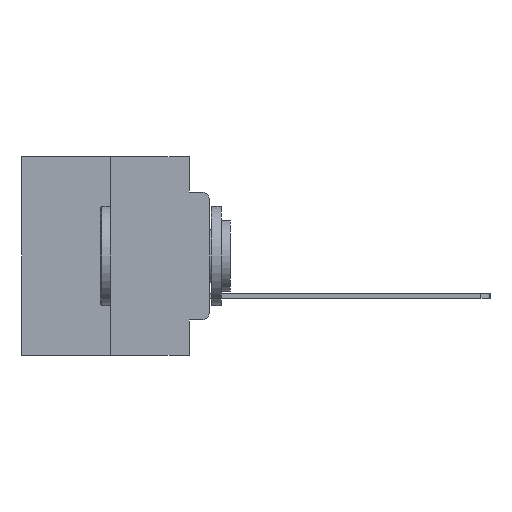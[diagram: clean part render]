
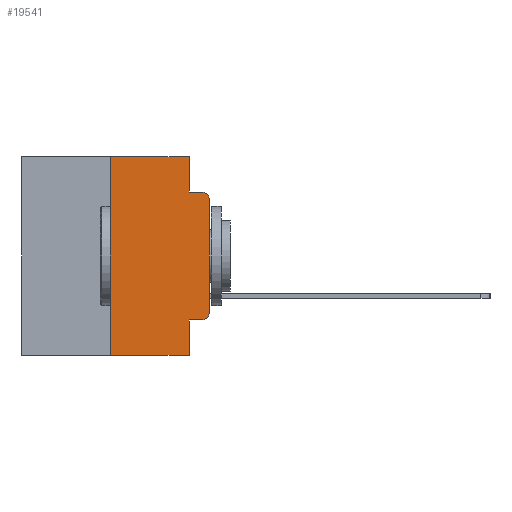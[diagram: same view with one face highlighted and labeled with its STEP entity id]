
A CAD part, left-side view. The second image highlights one B-rep face of the part: STEP entity #19541.
In plain terms, the highlighted planar face has unit normal (-1, 0, 0).
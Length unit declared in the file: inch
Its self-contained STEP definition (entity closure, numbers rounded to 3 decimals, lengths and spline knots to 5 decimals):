
#303 = VECTOR ( 'NONE', #25448, 39.37008 ) ;
#436 = CARTESIAN_POINT ( 'NONE',  ( 0., 0.473, 0. ) ) ;
#485 = ORIENTED_EDGE ( 'NONE', *, *, #19054, .T. ) ;
#502 = CARTESIAN_POINT ( 'NONE',  ( 0., 0.051, 0. ) ) ;
#745 = CARTESIAN_POINT ( 'NONE',  ( 0., 0.473, -0.5 ) ) ;
#862 = AXIS2_PLACEMENT_3D ( 'NONE', #10973, #25536, #13118 ) ;
#1314 = EDGE_CURVE ( 'NONE', #26206, #25900, #19107, .T. ) ;
#1725 = ORIENTED_EDGE ( 'NONE', *, *, #19400, .F. ) ;
#2042 = AXIS2_PLACEMENT_3D ( 'NONE', #21464, #8887, #23537 ) ;
#2920 = DIRECTION ( 'NONE',  ( 0., -1., 0. ) ) ;
#3387 = VECTOR ( 'NONE', #6915, 39.37008 ) ;
#3473 = CARTESIAN_POINT ( 'NONE',  ( 0., 0.051, -0.0885 ) ) ;
#3504 = VECTOR ( 'NONE', #16358, 39.37008 ) ;
#3799 = EDGE_CURVE ( 'NONE', #7085, #5451, #5358, .T. ) ;
#4054 = ORIENTED_EDGE ( 'NONE', *, *, #3799, .T. ) ;
#4371 = CARTESIAN_POINT ( 'NONE',  ( 0., 0.051, -0.4115 ) ) ;
#4598 = VERTEX_POINT ( 'NONE', #15596 ) ;
#5358 = LINE ( 'NONE', #16427, #16022 ) ;
#5361 = CIRCLE ( 'NONE', #862, 0.02 ) ;
#5451 = VERTEX_POINT ( 'NONE', #12956 ) ;
#6039 = VERTEX_POINT ( 'NONE', #6753 ) ;
#6254 = ORIENTED_EDGE ( 'NONE', *, *, #1314, .F. ) ;
#6753 = CARTESIAN_POINT ( 'NONE',  ( 0., 0.051, -0.0885 ) ) ;
#6915 = DIRECTION ( 'NONE',  ( 0., -1., 0. ) ) ;
#7085 = VERTEX_POINT ( 'NONE', #4371 ) ;
#8029 = VECTOR ( 'NONE', #9062, 39.37008 ) ;
#8144 = CARTESIAN_POINT ( 'NONE',  ( 0., 0.25, 0. ) ) ;
#8887 = DIRECTION ( 'NONE',  ( -1., 0., 0. ) ) ;
#9062 = DIRECTION ( 'NONE',  ( 0., 0., -1. ) ) ;
#9314 = LINE ( 'NONE', #745, #19206 ) ;
#9753 = LINE ( 'NONE', #436, #3387 ) ;
#9881 = EDGE_CURVE ( 'NONE', #4598, #6039, #19247, .T. ) ;
#9950 = CARTESIAN_POINT ( 'NONE',  ( 0., 0.02, -0.0885 ) ) ;
#10298 = VERTEX_POINT ( 'NONE', #17089 ) ;
#10390 = DIRECTION ( 'NONE',  ( 0., 0., -1. ) ) ;
#10875 = CARTESIAN_POINT ( 'NONE',  ( 0., 0., 0. ) ) ;
#10952 = ORIENTED_EDGE ( 'NONE', *, *, #19436, .F. ) ;
#10973 = CARTESIAN_POINT ( 'NONE',  ( 0., 0.02, -0.3915 ) ) ;
#11281 = CARTESIAN_POINT ( 'NONE',  ( 0., 0.25, -0.5 ) ) ;
#12907 = EDGE_CURVE ( 'NONE', #27122, #15659, #14839, .T. ) ;
#12956 = CARTESIAN_POINT ( 'NONE',  ( 0., 0.02, -0.4115 ) ) ;
#13118 = DIRECTION ( 'NONE',  ( 0., 0., -1. ) ) ;
#13703 = VECTOR ( 'NONE', #26496, 39.37008 ) ;
#14209 = EDGE_CURVE ( 'NONE', #26206, #10298, #9314, .T. ) ;
#14231 = CARTESIAN_POINT ( 'NONE',  ( 0., 0.051, 0. ) ) ;
#14839 = CIRCLE ( 'NONE', #2042, 0.02 ) ;
#15596 = CARTESIAN_POINT ( 'NONE',  ( 0., 0.051, 0. ) ) ;
#15659 = VERTEX_POINT ( 'NONE', #9950 ) ;
#16022 = VECTOR ( 'NONE', #24745, 39.37008 ) ;
#16358 = DIRECTION ( 'NONE',  ( 0., 0., 1. ) ) ;
#16427 = CARTESIAN_POINT ( 'NONE',  ( 0., 0.051, -0.4115 ) ) ;
#16537 = VERTEX_POINT ( 'NONE', #17227 ) ;
#16683 = CARTESIAN_POINT ( 'NONE',  ( 0., 0.473, 0. ) ) ;
#17089 = CARTESIAN_POINT ( 'NONE',  ( 0., 0.051, -0.5 ) ) ;
#17227 = CARTESIAN_POINT ( 'NONE',  ( 0., 0., -0.3915 ) ) ;
#17430 = CARTESIAN_POINT ( 'NONE',  ( 0., 0.25, 0. ) ) ;
#18614 = VECTOR ( 'NONE', #26595, 39.37008 ) ;
#18928 = ORIENTED_EDGE ( 'NONE', *, *, #12907, .T. ) ;
#19054 = EDGE_CURVE ( 'NONE', #16537, #27122, #22207, .T. ) ;
#19086 = EDGE_CURVE ( 'NONE', #5451, #16537, #5361, .T. ) ;
#19107 = LINE ( 'NONE', #17430, #3504 ) ;
#19206 = VECTOR ( 'NONE', #2920, 39.37008 ) ;
#19247 = LINE ( 'NONE', #502, #8029 ) ;
#19268 = LINE ( 'NONE', #3473, #13703 ) ;
#19400 = EDGE_CURVE ( 'NONE', #6039, #15659, #19268, .T. ) ;
#19436 = EDGE_CURVE ( 'NONE', #7085, #10298, #24106, .T. ) ;
#19541 = ADVANCED_FACE ( 'NONE', ( #26308 ), #20892, .F. ) ;
#19806 = EDGE_CURVE ( 'NONE', #25900, #4598, #9753, .T. ) ;
#20823 = ORIENTED_EDGE ( 'NONE', *, *, #14209, .T. ) ;
#20892 = PLANE ( 'NONE',  #23026 ) ;
#21240 = EDGE_LOOP ( 'NONE', ( #485, #18928, #1725, #22002, #23304, #6254, #20823, #10952, #4054, #23651 ) ) ;
#21464 = CARTESIAN_POINT ( 'NONE',  ( 0., 0.02, -0.1085 ) ) ;
#22002 = ORIENTED_EDGE ( 'NONE', *, *, #9881, .F. ) ;
#22207 = LINE ( 'NONE', #10875, #303 ) ;
#22953 = DIRECTION ( 'NONE',  ( 1., 0., 0. ) ) ;
#23026 = AXIS2_PLACEMENT_3D ( 'NONE', #16683, #22953, #10390 ) ;
#23304 = ORIENTED_EDGE ( 'NONE', *, *, #19806, .F. ) ;
#23537 = DIRECTION ( 'NONE',  ( 0., 0., -1. ) ) ;
#23651 = ORIENTED_EDGE ( 'NONE', *, *, #19086, .T. ) ;
#24106 = LINE ( 'NONE', #14231, #18614 ) ;
#24745 = DIRECTION ( 'NONE',  ( 0., -1., 0. ) ) ;
#25448 = DIRECTION ( 'NONE',  ( 0., 0., 1. ) ) ;
#25536 = DIRECTION ( 'NONE',  ( -1., 0., 0. ) ) ;
#25900 = VERTEX_POINT ( 'NONE', #8144 ) ;
#26206 = VERTEX_POINT ( 'NONE', #11281 ) ;
#26308 = FACE_OUTER_BOUND ( 'NONE', #21240, .T. ) ;
#26496 = DIRECTION ( 'NONE',  ( 0., -1., 0. ) ) ;
#26595 = DIRECTION ( 'NONE',  ( 0., 0., -1. ) ) ;
#26844 = CARTESIAN_POINT ( 'NONE',  ( 0., 0., -0.1085 ) ) ;
#27122 = VERTEX_POINT ( 'NONE', #26844 ) ;
